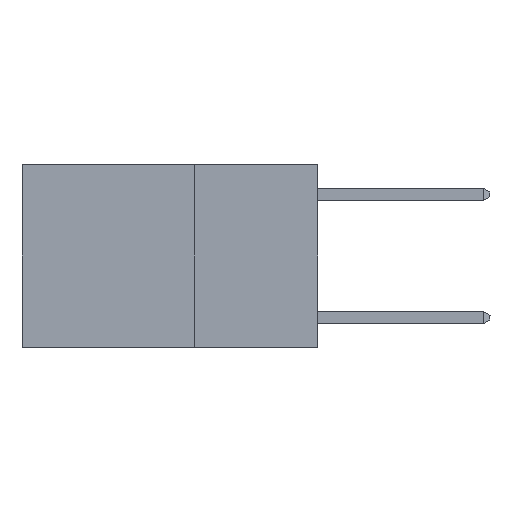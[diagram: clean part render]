
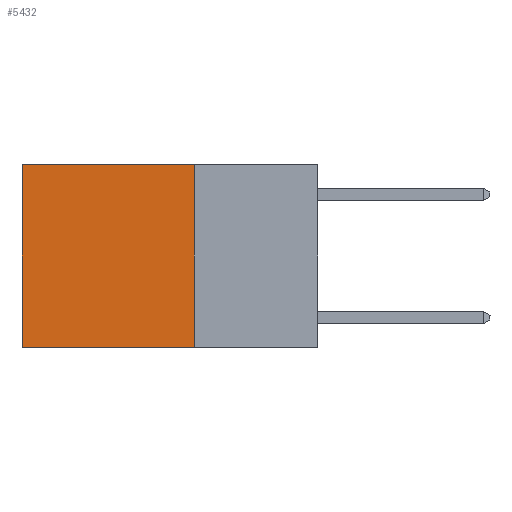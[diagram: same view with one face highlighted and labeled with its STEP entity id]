
A CAD part, left-side view. The second image highlights one B-rep face of the part: STEP entity #5432.
In plain terms, the highlighted planar face has unit normal (-1, 0, 0).
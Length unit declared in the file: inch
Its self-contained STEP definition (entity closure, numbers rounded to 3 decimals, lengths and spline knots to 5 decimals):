
#254 = ORIENTED_EDGE ( 'NONE', *, *, #3273, .T. ) ;
#262 = DIRECTION ( 'NONE',  ( 0., 1., 0. ) ) ;
#381 = LINE ( 'NONE', #4505, #7591 ) ;
#767 = CARTESIAN_POINT ( 'NONE',  ( 0.2625, 0.25, 0. ) ) ;
#1998 = ORIENTED_EDGE ( 'NONE', *, *, #14369, .F. ) ;
#2049 = CARTESIAN_POINT ( 'NONE',  ( 0.2625, 0.25, 0. ) ) ;
#2142 = LINE ( 'NONE', #767, #11811 ) ;
#2181 = ORIENTED_EDGE ( 'NONE', *, *, #10541, .F. ) ;
#3273 = EDGE_CURVE ( 'NONE', #5636, #7179, #12770, .T. ) ;
#4461 = LINE ( 'NONE', #17577, #11471 ) ;
#4505 = CARTESIAN_POINT ( 'NONE',  ( 0.2625, 0.25, 0. ) ) ;
#4747 = AXIS2_PLACEMENT_3D ( 'NONE', #2049, #17412, #11869 ) ;
#5432 = ADVANCED_FACE ( 'NONE', ( #13781 ), #17468, .F. ) ;
#5567 = CARTESIAN_POINT ( 'NONE',  ( 0.2625, 0.25, -0.37 ) ) ;
#5636 = VERTEX_POINT ( 'NONE', #17888 ) ;
#6122 = EDGE_CURVE ( 'NONE', #15055, #5636, #381, .T. ) ;
#7064 = VECTOR ( 'NONE', #11363, 39.37008 ) ;
#7179 = VERTEX_POINT ( 'NONE', #15399 ) ;
#7417 = ORIENTED_EDGE ( 'NONE', *, *, #6122, .T. ) ;
#7591 = VECTOR ( 'NONE', #262, 39.37008 ) ;
#10319 = EDGE_LOOP ( 'NONE', ( #254, #1998, #2181, #7417 ) ) ;
#10339 = CARTESIAN_POINT ( 'NONE',  ( 0.2625, 0.25, 0. ) ) ;
#10541 = EDGE_CURVE ( 'NONE', #15055, #12689, #2142, .T. ) ;
#10570 = DIRECTION ( 'NONE',  ( 0., 0., -1. ) ) ;
#11363 = DIRECTION ( 'NONE',  ( 0., 0., -1. ) ) ;
#11471 = VECTOR ( 'NONE', #11848, 39.37008 ) ;
#11811 = VECTOR ( 'NONE', #10570, 39.37008 ) ;
#11848 = DIRECTION ( 'NONE',  ( 0., 1., 0. ) ) ;
#11869 = DIRECTION ( 'NONE',  ( 0., 0., -1. ) ) ;
#12689 = VERTEX_POINT ( 'NONE', #5567 ) ;
#12770 = LINE ( 'NONE', #16725, #7064 ) ;
#13781 = FACE_OUTER_BOUND ( 'NONE', #10319, .T. ) ;
#14369 = EDGE_CURVE ( 'NONE', #12689, #7179, #4461, .T. ) ;
#15055 = VERTEX_POINT ( 'NONE', #10339 ) ;
#15399 = CARTESIAN_POINT ( 'NONE',  ( 0.2625, 0.6, -0.37 ) ) ;
#16725 = CARTESIAN_POINT ( 'NONE',  ( 0.2625, 0.6, 0. ) ) ;
#17412 = DIRECTION ( 'NONE',  ( 1., 0., 0. ) ) ;
#17468 = PLANE ( 'NONE',  #4747 ) ;
#17577 = CARTESIAN_POINT ( 'NONE',  ( 0.2625, 0.25, -0.37 ) ) ;
#17888 = CARTESIAN_POINT ( 'NONE',  ( 0.2625, 0.6, 0. ) ) ;
